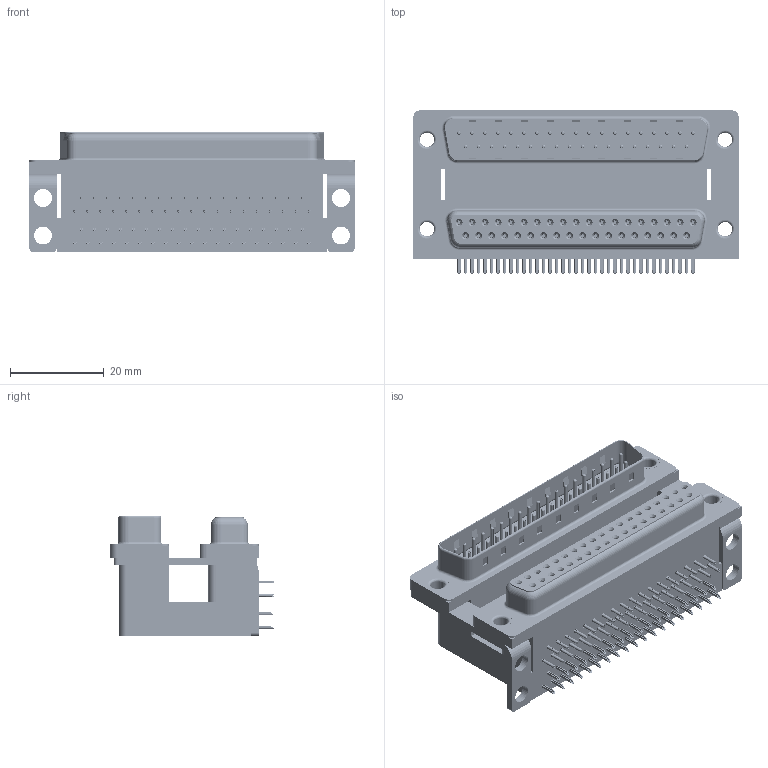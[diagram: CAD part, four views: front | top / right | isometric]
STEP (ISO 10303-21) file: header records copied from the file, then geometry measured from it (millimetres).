
FILE_DESCRIPTION (( 'STEP AP203' ), '1' );
FILE_NAME ('663-037-664-007.STEP', '2022-06-21T13:36:49', ( '' ), ( '' ), 'SwSTEP 2.0', 'SolidWorks 2020', '' );
FILE_SCHEMA (( 'CONFIG_CONTROL_DESIGN' ));
Length unit declared in the file: millimetre
Products named in the file (12): 663 Contact Top Lower; 663 Shell Plug_37 Contacts; 663 Thru Hole Rivet; 663 Shell Receptacle_37 Contacts; 663 Housing Spacer_37 Contacts M; 663 Contact Top Upper_M; 663 Housing Upper_37 Contacts M; 663 Housing Lower_37 Contacts; 663 Contact Bottom Lower; 663-037-664-007; 663 Mounting Bracket_NoneM; 663 Contact Bottom Upper_M
Assembly tree (85 placements, depth 2):
  663-037-664-007
    663 Housing Lower_37 Contacts
    663 Housing Spacer_37 Contacts M
    663 Housing Upper_37 Contacts M
    663 Shell Receptacle_37 Contacts
    663 Shell Plug_37 Contacts
    663 Contact Bottom Lower  x18
    663 Contact Top Lower  x19
    663 Contact Bottom Upper_M  x18
    663 Contact Top Upper_M  x19
    663 Mounting Bracket_NoneM  x2
    663 Thru Hole Rivet  x4
Bounding box: 69.32 x 34.78 x 25.6 mm (x, y, z)
Volume: 31176.6 mm3; surface area: 32298 mm2
Topology: 85 solids, 85 shells, 8861 faces, 22793 edges, 14221 vertices
Faces by surface type: plane 4741, cylinder 2141, bspline 1260, cone 444, torus 275
Entity records: 65155 total; most frequent: CARTESIAN_POINT 13856, ORIENTED_EDGE 9902, DIRECTION 9586, EDGE_CURVE 4951, VECTOR 3770, LINE 3770, VERTEX_POINT 3193, AXIS2_PLACEMENT_3D 2908
